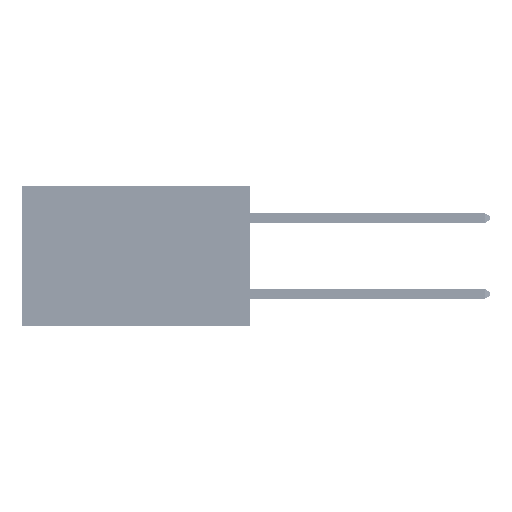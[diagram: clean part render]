
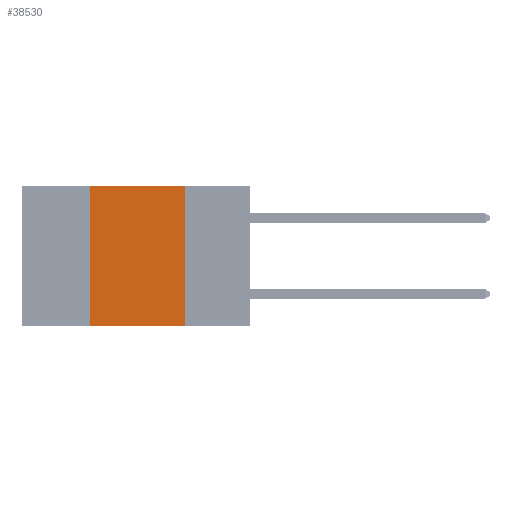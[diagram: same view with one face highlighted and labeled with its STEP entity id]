
A CAD part, left-side view. The second image highlights one B-rep face of the part: STEP entity #38530.
In plain terms, the highlighted planar face has unit normal (-1, 0, 0).
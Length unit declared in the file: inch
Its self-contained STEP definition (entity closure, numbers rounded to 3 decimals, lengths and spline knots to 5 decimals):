
#764 = VECTOR ( 'NONE', #4179, 39.37008 ) ;
#3917 = LINE ( 'NONE', #8154, #764 ) ;
#4179 = DIRECTION ( 'NONE',  ( 0., -1., 0. ) ) ;
#8154 = CARTESIAN_POINT ( 'NONE',  ( 0., 0.6, -0.37 ) ) ;
#9605 = ORIENTED_EDGE ( 'NONE', *, *, #22210, .T. ) ;
#10304 = VECTOR ( 'NONE', #23056, 39.37008 ) ;
#10579 = AXIS2_PLACEMENT_3D ( 'NONE', #31067, #42978, #22848 ) ;
#11958 = EDGE_CURVE ( 'NONE', #38215, #13987, #37500, .T. ) ;
#13987 = VERTEX_POINT ( 'NONE', #28198 ) ;
#14829 = CARTESIAN_POINT ( 'NONE',  ( 0., 0.6, 0. ) ) ;
#15890 = FACE_OUTER_BOUND ( 'NONE', #46134, .T. ) ;
#16144 = PLANE ( 'NONE',  #10579 ) ;
#17639 = VECTOR ( 'NONE', #29275, 39.37008 ) ;
#18204 = CARTESIAN_POINT ( 'NONE',  ( 0., 0.42, 0. ) ) ;
#18285 = EDGE_CURVE ( 'NONE', #33939, #38215, #32915, .T. ) ;
#19091 = LINE ( 'NONE', #27030, #10304 ) ;
#22210 = EDGE_CURVE ( 'NONE', #33939, #36027, #3917, .T. ) ;
#22420 = DIRECTION ( 'NONE',  ( 0., 0., 1. ) ) ;
#22848 = DIRECTION ( 'NONE',  ( 0., 0., -1. ) ) ;
#23056 = DIRECTION ( 'NONE',  ( 0., 0., -1. ) ) ;
#25817 = ORIENTED_EDGE ( 'NONE', *, *, #18285, .F. ) ;
#26615 = CARTESIAN_POINT ( 'NONE',  ( 0., 0.42, -0.37 ) ) ;
#27030 = CARTESIAN_POINT ( 'NONE',  ( 0., 0.17, 0. ) ) ;
#28198 = CARTESIAN_POINT ( 'NONE',  ( 0., 0.17, 0. ) ) ;
#29275 = DIRECTION ( 'NONE',  ( 0., -1., 0. ) ) ;
#31067 = CARTESIAN_POINT ( 'NONE',  ( 0., 0.6, 0. ) ) ;
#31220 = EDGE_CURVE ( 'NONE', #13987, #36027, #19091, .T. ) ;
#32117 = CARTESIAN_POINT ( 'NONE',  ( 0., 0.42, 0. ) ) ;
#32915 = LINE ( 'NONE', #18204, #43543 ) ;
#33939 = VERTEX_POINT ( 'NONE', #26615 ) ;
#36027 = VERTEX_POINT ( 'NONE', #43636 ) ;
#36327 = ORIENTED_EDGE ( 'NONE', *, *, #11958, .F. ) ;
#37500 = LINE ( 'NONE', #14829, #17639 ) ;
#38215 = VERTEX_POINT ( 'NONE', #32117 ) ;
#38530 = ADVANCED_FACE ( 'NONE', ( #15890 ), #16144, .F. ) ;
#42978 = DIRECTION ( 'NONE',  ( 1., 0., 0. ) ) ;
#43465 = ORIENTED_EDGE ( 'NONE', *, *, #31220, .F. ) ;
#43543 = VECTOR ( 'NONE', #22420, 39.37008 ) ;
#43636 = CARTESIAN_POINT ( 'NONE',  ( 0., 0.17, -0.37 ) ) ;
#46134 = EDGE_LOOP ( 'NONE', ( #43465, #36327, #25817, #9605 ) ) ;
